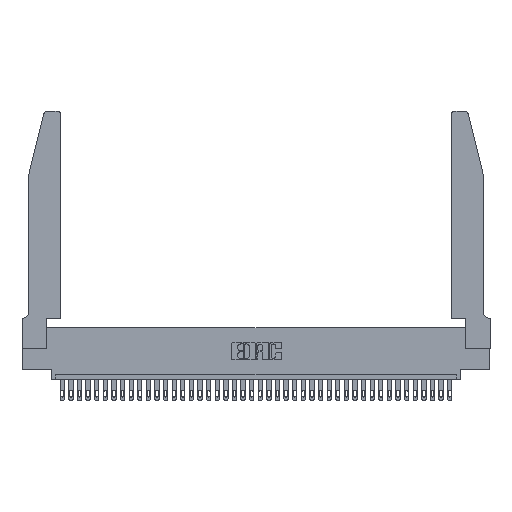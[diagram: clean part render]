
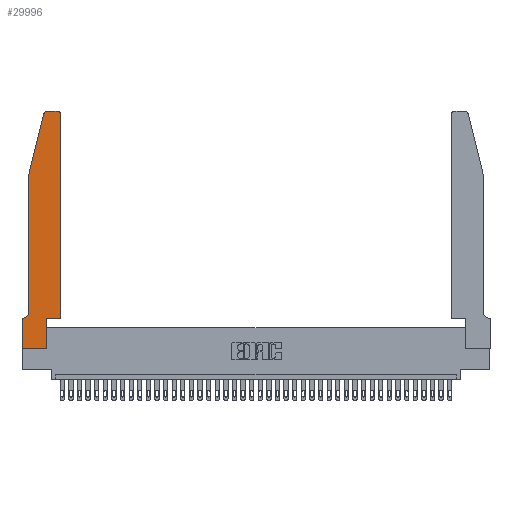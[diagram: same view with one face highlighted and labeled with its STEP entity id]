
A CAD part, top view. The second image highlights one B-rep face of the part: STEP entity #29996.
In plain terms, the highlighted planar face has unit normal (0, 0, 1).
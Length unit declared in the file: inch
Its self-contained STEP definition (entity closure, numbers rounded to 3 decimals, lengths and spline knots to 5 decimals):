
#99 = DIRECTION ( 'NONE',  ( 1., 0., 0. ) ) ;
#395 = CIRCLE ( 'NONE', #34604, 0.07 ) ;
#1512 = VERTEX_POINT ( 'NONE', #28473 ) ;
#3176 = ORIENTED_EDGE ( 'NONE', *, *, #11923, .T. ) ;
#3622 = CARTESIAN_POINT ( 'NONE',  ( 0.2865, 0., 0.37 ) ) ;
#3840 = CARTESIAN_POINT ( 'NONE',  ( 0.0755, 0.35, 0.37 ) ) ;
#4676 = AXIS2_PLACEMENT_3D ( 'NONE', #19503, #10739, #22550 ) ;
#4827 = VECTOR ( 'NONE', #37355, 39.37008 ) ;
#5156 = LINE ( 'NONE', #23424, #37086 ) ;
#5402 = DIRECTION ( 'NONE',  ( -1., 0., 0. ) ) ;
#6640 = ORIENTED_EDGE ( 'NONE', *, *, #17063, .T. ) ;
#6652 = VERTEX_POINT ( 'NONE', #34325 ) ;
#6707 = CARTESIAN_POINT ( 'NONE',  ( 0.284, 2.75, 0.37 ) ) ;
#6912 = DIRECTION ( 'NONE',  ( 0., -1., 0. ) ) ;
#7568 = VERTEX_POINT ( 'NONE', #11978 ) ;
#7628 = CARTESIAN_POINT ( 'NONE',  ( 0.25487, 2.72718, 0.37 ) ) ;
#7746 = CARTESIAN_POINT ( 'NONE',  ( 0.4505, 2.72, 0.37 ) ) ;
#8408 = EDGE_CURVE ( 'NONE', #1512, #7568, #32614, .T. ) ;
#8913 = DIRECTION ( 'NONE',  ( 0., 0., 1. ) ) ;
#8942 = CARTESIAN_POINT ( 'NONE',  ( 0.4205, 2.72, 0.37 ) ) ;
#9489 = AXIS2_PLACEMENT_3D ( 'NONE', #32707, #8913, #26361 ) ;
#9650 = DIRECTION ( 'NONE',  ( 1., 0., 0. ) ) ;
#9879 = LINE ( 'NONE', #25188, #14607 ) ;
#9908 = ORIENTED_EDGE ( 'NONE', *, *, #8408, .T. ) ;
#10373 = CARTESIAN_POINT ( 'NONE',  ( 0., 0., 0.37 ) ) ;
#10642 = ORIENTED_EDGE ( 'NONE', *, *, #37436, .T. ) ;
#10687 = EDGE_CURVE ( 'NONE', #16382, #6652, #20467, .T. ) ;
#10739 = DIRECTION ( 'NONE',  ( 0., 0., 1. ) ) ;
#10892 = DIRECTION ( 'NONE',  ( 1., 0., 0. ) ) ;
#10939 = LINE ( 'NONE', #16052, #4827 ) ;
#11045 = EDGE_CURVE ( 'NONE', #24091, #16382, #30768, .T. ) ;
#11923 = EDGE_CURVE ( 'NONE', #14890, #24091, #26496, .T. ) ;
#11978 = CARTESIAN_POINT ( 'NONE',  ( 0., 0.35, 0.37 ) ) ;
#12429 = VECTOR ( 'NONE', #9650, 39.37008 ) ;
#12521 = ORIENTED_EDGE ( 'NONE', *, *, #27483, .T. ) ;
#12842 = CARTESIAN_POINT ( 'NONE',  ( 0.0755, 2., 0.37 ) ) ;
#13325 = EDGE_CURVE ( 'NONE', #7568, #14890, #29244, .T. ) ;
#14607 = VECTOR ( 'NONE', #16504, 39.37008 ) ;
#14664 = CARTESIAN_POINT ( 'NONE',  ( 0., 0., 0.37 ) ) ;
#14890 = VERTEX_POINT ( 'NONE', #14664 ) ;
#15729 = DIRECTION ( 'NONE',  ( -1., 0., 0. ) ) ;
#16052 = CARTESIAN_POINT ( 'NONE',  ( 0.4505, 0.35, 0.37 ) ) ;
#16220 = ORIENTED_EDGE ( 'NONE', *, *, #13325, .T. ) ;
#16382 = VERTEX_POINT ( 'NONE', #19478 ) ;
#16504 = DIRECTION ( 'NONE',  ( 0., -1., 0. ) ) ;
#16881 = DIRECTION ( 'NONE',  ( 0., 1., 0. ) ) ;
#17024 = VERTEX_POINT ( 'NONE', #25311 ) ;
#17063 = EDGE_CURVE ( 'NONE', #17024, #19380, #9879, .T. ) ;
#17292 = PLANE ( 'NONE',  #9489 ) ;
#17718 = CIRCLE ( 'NONE', #32857, 0.03 ) ;
#18475 = VECTOR ( 'NONE', #10892, 39.37008 ) ;
#18660 = CARTESIAN_POINT ( 'NONE',  ( 0., 0., 0.37 ) ) ;
#18873 = LINE ( 'NONE', #12842, #26900 ) ;
#19380 = VERTEX_POINT ( 'NONE', #36259 ) ;
#19478 = CARTESIAN_POINT ( 'NONE',  ( 0.2865, 0.35, 0.37 ) ) ;
#19503 = CARTESIAN_POINT ( 'NONE',  ( 0.284, 2.72, 0.37 ) ) ;
#20467 = LINE ( 'NONE', #35954, #12429 ) ;
#20487 = EDGE_CURVE ( 'NONE', #29696, #29818, #32675, .T. ) ;
#20498 = ORIENTED_EDGE ( 'NONE', *, *, #10687, .T. ) ;
#21217 = VECTOR ( 'NONE', #6912, 39.37008 ) ;
#22550 = DIRECTION ( 'NONE',  ( 1., 0., 0. ) ) ;
#23424 = CARTESIAN_POINT ( 'NONE',  ( 0.2605, 2.75, 0.37 ) ) ;
#24091 = VERTEX_POINT ( 'NONE', #3622 ) ;
#24580 = ORIENTED_EDGE ( 'NONE', *, *, #20487, .T. ) ;
#24818 = DIRECTION ( 'NONE',  ( 0., 0., -1. ) ) ;
#24858 = DIRECTION ( 'NONE',  ( -1., 0., 0. ) ) ;
#25188 = CARTESIAN_POINT ( 'NONE',  ( 0.0755, 2., 0.37 ) ) ;
#25311 = CARTESIAN_POINT ( 'NONE',  ( 0.0755, 2., 0.37 ) ) ;
#25807 = EDGE_LOOP ( 'NONE', ( #10642, #24580, #12521, #6640, #35532, #9908, #16220, #3176, #26563, #20498, #35737, #34979 ) ) ;
#26361 = DIRECTION ( 'NONE',  ( 1., 0., 0. ) ) ;
#26496 = LINE ( 'NONE', #10373, #18475 ) ;
#26563 = ORIENTED_EDGE ( 'NONE', *, *, #11045, .T. ) ;
#26900 = VECTOR ( 'NONE', #36901, 39.37008 ) ;
#27194 = FACE_OUTER_BOUND ( 'NONE', #25807, .T. ) ;
#27483 = EDGE_CURVE ( 'NONE', #29818, #17024, #18873, .T. ) ;
#27577 = CARTESIAN_POINT ( 'NONE',  ( 0.0055, 0.42, 0.37 ) ) ;
#28473 = CARTESIAN_POINT ( 'NONE',  ( 0.0055, 0.35, 0.37 ) ) ;
#29244 = LINE ( 'NONE', #18660, #21217 ) ;
#29289 = VERTEX_POINT ( 'NONE', #38488 ) ;
#29300 = VECTOR ( 'NONE', #24858, 39.37008 ) ;
#29611 = EDGE_CURVE ( 'NONE', #19380, #1512, #395, .T. ) ;
#29696 = VERTEX_POINT ( 'NONE', #6707 ) ;
#29818 = VERTEX_POINT ( 'NONE', #7628 ) ;
#29996 = ADVANCED_FACE ( 'NONE', ( #27194 ), #17292, .T. ) ;
#30768 = LINE ( 'NONE', #38177, #34492 ) ;
#32614 = LINE ( 'NONE', #3840, #29300 ) ;
#32675 = CIRCLE ( 'NONE', #4676, 0.03 ) ;
#32707 = CARTESIAN_POINT ( 'NONE',  ( 0., 0.35, 0.37 ) ) ;
#32857 = AXIS2_PLACEMENT_3D ( 'NONE', #8942, #36341, #99 ) ;
#33169 = EDGE_CURVE ( 'NONE', #6652, #37949, #10939, .T. ) ;
#34325 = CARTESIAN_POINT ( 'NONE',  ( 0.4505, 0.35, 0.37 ) ) ;
#34492 = VECTOR ( 'NONE', #16881, 39.37008 ) ;
#34604 = AXIS2_PLACEMENT_3D ( 'NONE', #27577, #24818, #15729 ) ;
#34979 = ORIENTED_EDGE ( 'NONE', *, *, #38827, .T. ) ;
#35532 = ORIENTED_EDGE ( 'NONE', *, *, #29611, .T. ) ;
#35737 = ORIENTED_EDGE ( 'NONE', *, *, #33169, .T. ) ;
#35954 = CARTESIAN_POINT ( 'NONE',  ( 0.4505, 0.35, 0.37 ) ) ;
#36259 = CARTESIAN_POINT ( 'NONE',  ( 0.0755, 0.42, 0.37 ) ) ;
#36341 = DIRECTION ( 'NONE',  ( 0., 0., 1. ) ) ;
#36901 = DIRECTION ( 'NONE',  ( -0.239, -0.971, 0. ) ) ;
#37086 = VECTOR ( 'NONE', #5402, 39.37008 ) ;
#37355 = DIRECTION ( 'NONE',  ( 0., 1., 0. ) ) ;
#37436 = EDGE_CURVE ( 'NONE', #29289, #29696, #5156, .T. ) ;
#37949 = VERTEX_POINT ( 'NONE', #7746 ) ;
#38177 = CARTESIAN_POINT ( 'NONE',  ( 0.2865, 0.35, 0.37 ) ) ;
#38488 = CARTESIAN_POINT ( 'NONE',  ( 0.4205, 2.75, 0.37 ) ) ;
#38827 = EDGE_CURVE ( 'NONE', #37949, #29289, #17718, .T. ) ;
